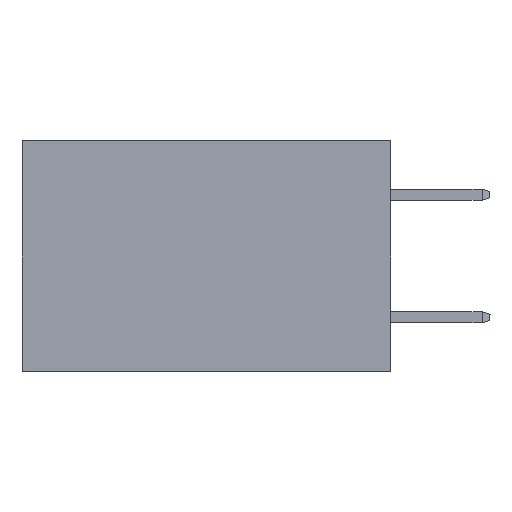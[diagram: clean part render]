
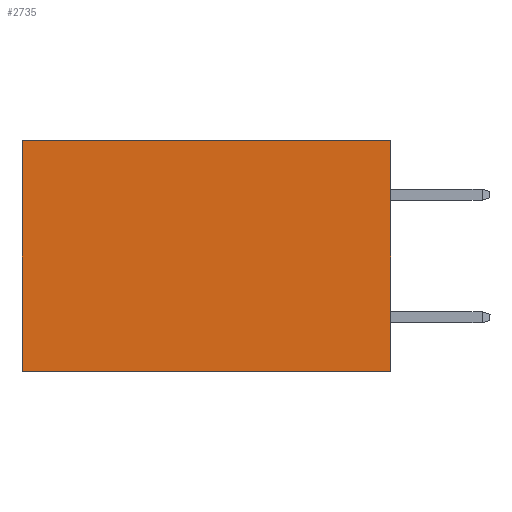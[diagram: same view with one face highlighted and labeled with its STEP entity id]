
A CAD part, left-side view. The second image highlights one B-rep face of the part: STEP entity #2735.
In plain terms, the highlighted planar face has unit normal (-1, 0, 0).
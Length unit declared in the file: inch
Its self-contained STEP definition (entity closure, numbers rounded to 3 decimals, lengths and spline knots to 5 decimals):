
#465 = DIRECTION ( 'NONE',  ( 1., 0., 0. ) ) ;
#689 = CARTESIAN_POINT ( 'NONE',  ( 0.2875, 0., 0. ) ) ;
#902 = FACE_OUTER_BOUND ( 'NONE', #12528, .T. ) ;
#927 = DIRECTION ( 'NONE',  ( 0., 1., 0. ) ) ;
#2118 = VERTEX_POINT ( 'NONE', #689 ) ;
#2735 = ADVANCED_FACE ( 'NONE', ( #902 ), #14970, .F. ) ;
#2970 = VERTEX_POINT ( 'NONE', #14250 ) ;
#3058 = EDGE_CURVE ( 'NONE', #5464, #15821, #14409, .T. ) ;
#3382 = VECTOR ( 'NONE', #17169, 39.37008 ) ;
#3820 = ORIENTED_EDGE ( 'NONE', *, *, #3058, .F. ) ;
#4562 = AXIS2_PLACEMENT_3D ( 'NONE', #16402, #465, #17892 ) ;
#4757 = LINE ( 'NONE', #14114, #7220 ) ;
#5464 = VERTEX_POINT ( 'NONE', #8057 ) ;
#5842 = LINE ( 'NONE', #9825, #3382 ) ;
#6961 = VECTOR ( 'NONE', #927, 39.37008 ) ;
#7220 = VECTOR ( 'NONE', #14170, 39.37008 ) ;
#8057 = CARTESIAN_POINT ( 'NONE',  ( 0.2875, 0., -0.375 ) ) ;
#9183 = ORIENTED_EDGE ( 'NONE', *, *, #13767, .T. ) ;
#9825 = CARTESIAN_POINT ( 'NONE',  ( 0.2875, 0., -0.375 ) ) ;
#10867 = LINE ( 'NONE', #18419, #15615 ) ;
#12411 = ORIENTED_EDGE ( 'NONE', *, *, #12773, .T. ) ;
#12528 = EDGE_LOOP ( 'NONE', ( #9183, #3820, #13016, #12411 ) ) ;
#12773 = EDGE_CURVE ( 'NONE', #2118, #2970, #10867, .T. ) ;
#13016 = ORIENTED_EDGE ( 'NONE', *, *, #18237, .F. ) ;
#13767 = EDGE_CURVE ( 'NONE', #2970, #15821, #4757, .T. ) ;
#14114 = CARTESIAN_POINT ( 'NONE',  ( 0.2875, 0.6, -0.375 ) ) ;
#14170 = DIRECTION ( 'NONE',  ( 0., 0., -1. ) ) ;
#14250 = CARTESIAN_POINT ( 'NONE',  ( 0.2875, 0.6, 0. ) ) ;
#14359 = CARTESIAN_POINT ( 'NONE',  ( 0.2875, 0.6, -0.375 ) ) ;
#14409 = LINE ( 'NONE', #15108, #6961 ) ;
#14970 = PLANE ( 'NONE',  #4562 ) ;
#15108 = CARTESIAN_POINT ( 'NONE',  ( 0.2875, 0., -0.375 ) ) ;
#15615 = VECTOR ( 'NONE', #16926, 39.37008 ) ;
#15821 = VERTEX_POINT ( 'NONE', #14359 ) ;
#16402 = CARTESIAN_POINT ( 'NONE',  ( 0.2875, 0., -0.375 ) ) ;
#16926 = DIRECTION ( 'NONE',  ( 0., 1., 0. ) ) ;
#17169 = DIRECTION ( 'NONE',  ( 0., 0., -1. ) ) ;
#17892 = DIRECTION ( 'NONE',  ( 0., 0., -1. ) ) ;
#18237 = EDGE_CURVE ( 'NONE', #2118, #5464, #5842, .T. ) ;
#18419 = CARTESIAN_POINT ( 'NONE',  ( 0.2875, 0., 0. ) ) ;
